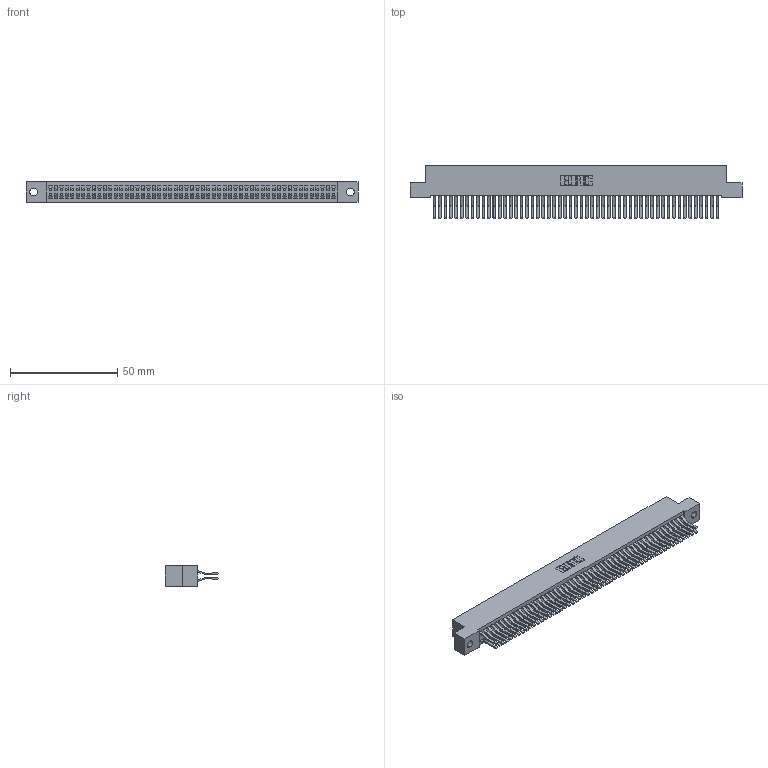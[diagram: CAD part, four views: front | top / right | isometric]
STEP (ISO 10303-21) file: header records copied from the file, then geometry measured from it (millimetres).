
FILE_DESCRIPTION (( 'STEP AP203' ), '1' );
FILE_NAME ('392-106-560-202.STEP', '2018-08-18T20:40:12', ( '' ), ( '' ), 'SwSTEP 2.0', 'SolidWorks 2016', '' );
FILE_SCHEMA (( 'CONFIG_CONTROL_DESIGN' ));
Length unit declared in the file: inch
Products named in the file (3): 342 Part_.128 Slot; 345-292-001_560 Tail; 392-106-560-202
Assembly tree (107 placements, depth 2):
  392-106-560-202
    342 Part_.128 Slot
    345-292-001_560 Tail  x106
Bounding box: 154.94 x 24.78 x 9.4 mm (x, y, z)
Volume: 14617.2 mm3; surface area: 25492.4 mm2
Topology: 107 solids, 107 shells, 5838 faces, 17377 edges, 11442 vertices
Faces by surface type: plane 3886, cylinder 1952
Entity records: 32765 total; most frequent: CARTESIAN_POINT 5418, ORIENTED_EDGE 5354, DIRECTION 4613, EDGE_CURVE 2677, VECTOR 2545, LINE 2545, VERTEX_POINT 1782, AXIS2_PLACEMENT_3D 1034
